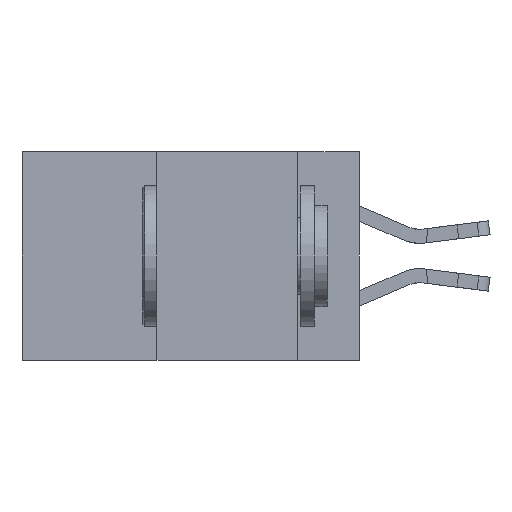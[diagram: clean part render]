
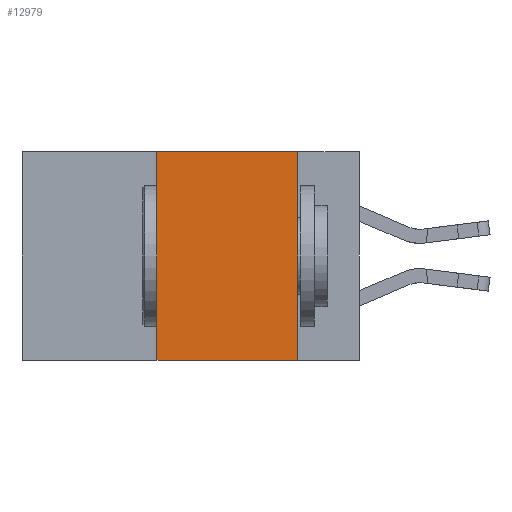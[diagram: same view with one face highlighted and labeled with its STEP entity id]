
A CAD part, left-side view. The second image highlights one B-rep face of the part: STEP entity #12979.
In plain terms, the highlighted planar face has unit normal (-1, 0, 0).
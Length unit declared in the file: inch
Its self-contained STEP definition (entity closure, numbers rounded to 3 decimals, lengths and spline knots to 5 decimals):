
#1306 = LINE ( 'NONE', #14843, #25235 ) ;
#2503 = DIRECTION ( 'NONE',  ( 0., 0., -1. ) ) ;
#2699 = VECTOR ( 'NONE', #19757, 39.37008 ) ;
#3100 = VERTEX_POINT ( 'NONE', #16035 ) ;
#3770 = EDGE_CURVE ( 'NONE', #6763, #15860, #1306, .T. ) ;
#4839 = LINE ( 'NONE', #11563, #2699 ) ;
#6288 = VECTOR ( 'NONE', #25225, 39.37008 ) ;
#6763 = VERTEX_POINT ( 'NONE', #20083 ) ;
#9629 = ORIENTED_EDGE ( 'NONE', *, *, #3770, .F. ) ;
#10311 = AXIS2_PLACEMENT_3D ( 'NONE', #29091, #21128, #2503 ) ;
#10412 = ORIENTED_EDGE ( 'NONE', *, *, #13129, .F. ) ;
#11563 = CARTESIAN_POINT ( 'NONE',  ( 0., 0.6, -0.37 ) ) ;
#11740 = CARTESIAN_POINT ( 'NONE',  ( 0., 0.6, 0. ) ) ;
#11780 = CARTESIAN_POINT ( 'NONE',  ( 0., 0.36, 0. ) ) ;
#12979 = ADVANCED_FACE ( 'NONE', ( #27698 ), #15971, .F. ) ;
#13129 = EDGE_CURVE ( 'NONE', #28321, #6763, #20929, .T. ) ;
#13866 = CARTESIAN_POINT ( 'NONE',  ( 0., 0.11, -0.37 ) ) ;
#14843 = CARTESIAN_POINT ( 'NONE',  ( 0., 0.11, 0. ) ) ;
#15860 = VERTEX_POINT ( 'NONE', #13866 ) ;
#15971 = PLANE ( 'NONE',  #10311 ) ;
#16035 = CARTESIAN_POINT ( 'NONE',  ( 0., 0.36, -0.37 ) ) ;
#17086 = DIRECTION ( 'NONE',  ( 0., 0., -1. ) ) ;
#18013 = VECTOR ( 'NONE', #20273, 39.37008 ) ;
#19757 = DIRECTION ( 'NONE',  ( 0., -1., 0. ) ) ;
#20083 = CARTESIAN_POINT ( 'NONE',  ( 0., 0.11, 0. ) ) ;
#20273 = DIRECTION ( 'NONE',  ( 0., 0., 1. ) ) ;
#20929 = LINE ( 'NONE', #11740, #6288 ) ;
#21128 = DIRECTION ( 'NONE',  ( 1., 0., 0. ) ) ;
#21657 = ORIENTED_EDGE ( 'NONE', *, *, #29052, .F. ) ;
#22883 = CARTESIAN_POINT ( 'NONE',  ( 0., 0.36, 0. ) ) ;
#25225 = DIRECTION ( 'NONE',  ( 0., -1., 0. ) ) ;
#25235 = VECTOR ( 'NONE', #17086, 39.37008 ) ;
#26689 = EDGE_LOOP ( 'NONE', ( #9629, #10412, #21657, #26866 ) ) ;
#26866 = ORIENTED_EDGE ( 'NONE', *, *, #33707, .T. ) ;
#27698 = FACE_OUTER_BOUND ( 'NONE', #26689, .T. ) ;
#28321 = VERTEX_POINT ( 'NONE', #11780 ) ;
#29052 = EDGE_CURVE ( 'NONE', #3100, #28321, #31012, .T. ) ;
#29091 = CARTESIAN_POINT ( 'NONE',  ( 0., 0.6, 0. ) ) ;
#31012 = LINE ( 'NONE', #22883, #18013 ) ;
#33707 = EDGE_CURVE ( 'NONE', #3100, #15860, #4839, .T. ) ;
